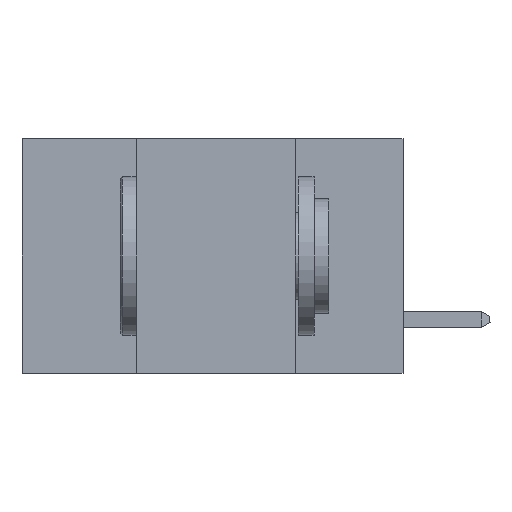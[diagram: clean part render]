
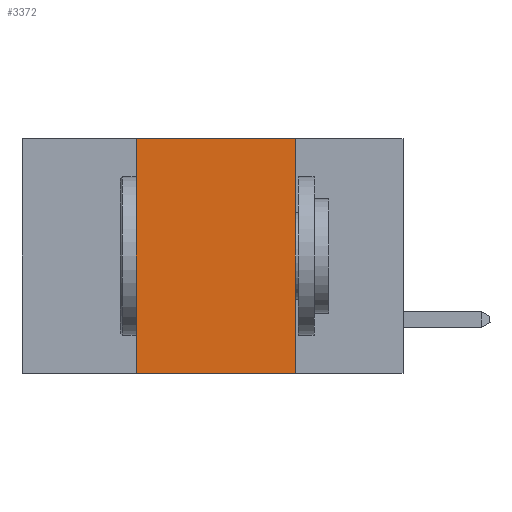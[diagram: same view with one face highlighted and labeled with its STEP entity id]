
A CAD part, left-side view. The second image highlights one B-rep face of the part: STEP entity #3372.
In plain terms, the highlighted planar face has unit normal (-1, 0, 0).
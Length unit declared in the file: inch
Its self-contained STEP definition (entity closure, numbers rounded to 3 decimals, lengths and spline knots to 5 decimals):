
#402 = DIRECTION ( 'NONE',  ( 1., 0., 0. ) ) ;
#3305 = DIRECTION ( 'NONE',  ( 0., 0., -1. ) ) ;
#3372 = ADVANCED_FACE ( 'NONE', ( #20497 ), #17862, .F. ) ;
#3538 = EDGE_CURVE ( 'NONE', #16048, #33044, #35198, .T. ) ;
#3733 = VERTEX_POINT ( 'NONE', #19207 ) ;
#3758 = AXIS2_PLACEMENT_3D ( 'NONE', #8940, #402, #3305 ) ;
#4377 = ORIENTED_EDGE ( 'NONE', *, *, #10664, .F. ) ;
#6919 = LINE ( 'NONE', #22065, #29977 ) ;
#7573 = CARTESIAN_POINT ( 'NONE',  ( 0., 0.42, -0.37 ) ) ;
#8940 = CARTESIAN_POINT ( 'NONE',  ( 0., 0.6, 0. ) ) ;
#9685 = CARTESIAN_POINT ( 'NONE',  ( 0., 0.42, 0. ) ) ;
#10227 = VERTEX_POINT ( 'NONE', #33609 ) ;
#10471 = CARTESIAN_POINT ( 'NONE',  ( 0., 0.17, 0. ) ) ;
#10664 = EDGE_CURVE ( 'NONE', #33044, #10227, #6919, .T. ) ;
#11633 = DIRECTION ( 'NONE',  ( 0., 0., -1. ) ) ;
#13928 = CARTESIAN_POINT ( 'NONE',  ( 0., 0.6, -0.37 ) ) ;
#15168 = LINE ( 'NONE', #10471, #24494 ) ;
#15856 = DIRECTION ( 'NONE',  ( 0., 0., 1. ) ) ;
#16048 = VERTEX_POINT ( 'NONE', #7573 ) ;
#17131 = EDGE_LOOP ( 'NONE', ( #28473, #4377, #36739, #23963 ) ) ;
#17862 = PLANE ( 'NONE',  #3758 ) ;
#19207 = CARTESIAN_POINT ( 'NONE',  ( 0., 0.17, -0.37 ) ) ;
#19350 = VECTOR ( 'NONE', #15856, 39.37008 ) ;
#20497 = FACE_OUTER_BOUND ( 'NONE', #17131, .T. ) ;
#22065 = CARTESIAN_POINT ( 'NONE',  ( 0., 0.6, 0. ) ) ;
#23948 = EDGE_CURVE ( 'NONE', #10227, #3733, #15168, .T. ) ;
#23963 = ORIENTED_EDGE ( 'NONE', *, *, #25416, .T. ) ;
#24494 = VECTOR ( 'NONE', #11633, 39.37008 ) ;
#25280 = DIRECTION ( 'NONE',  ( 0., -1., 0. ) ) ;
#25416 = EDGE_CURVE ( 'NONE', #16048, #3733, #33651, .T. ) ;
#26111 = VECTOR ( 'NONE', #25280, 39.37008 ) ;
#28473 = ORIENTED_EDGE ( 'NONE', *, *, #23948, .F. ) ;
#29977 = VECTOR ( 'NONE', #33119, 39.37008 ) ;
#31936 = CARTESIAN_POINT ( 'NONE',  ( 0., 0.42, 0. ) ) ;
#33044 = VERTEX_POINT ( 'NONE', #9685 ) ;
#33119 = DIRECTION ( 'NONE',  ( 0., -1., 0. ) ) ;
#33609 = CARTESIAN_POINT ( 'NONE',  ( 0., 0.17, 0. ) ) ;
#33651 = LINE ( 'NONE', #13928, #26111 ) ;
#35198 = LINE ( 'NONE', #31936, #19350 ) ;
#36739 = ORIENTED_EDGE ( 'NONE', *, *, #3538, .F. ) ;
